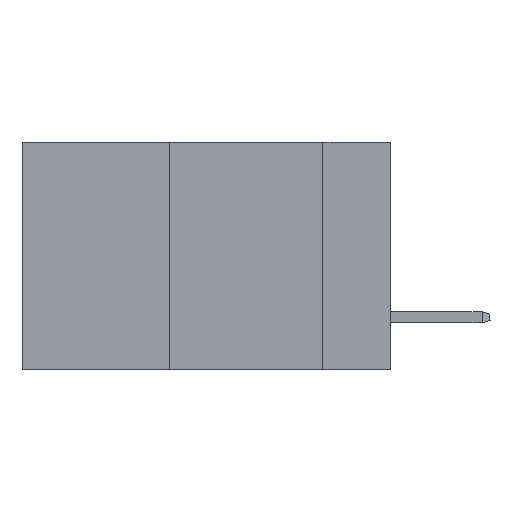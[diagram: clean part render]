
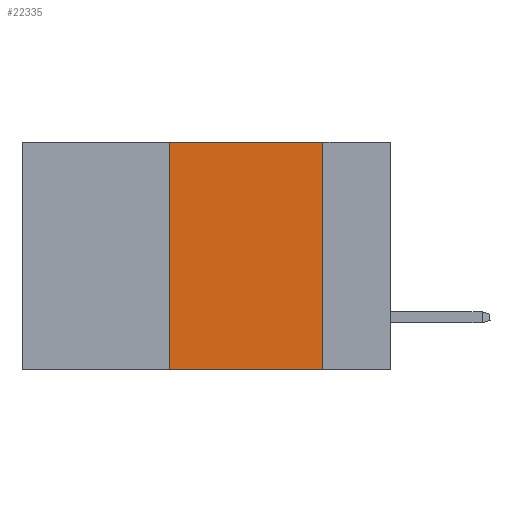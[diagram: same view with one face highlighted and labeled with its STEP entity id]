
A CAD part, left-side view. The second image highlights one B-rep face of the part: STEP entity #22335.
In plain terms, the highlighted planar face has unit normal (-1, 0, 0).
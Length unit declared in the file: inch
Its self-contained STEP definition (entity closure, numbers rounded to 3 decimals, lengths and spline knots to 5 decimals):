
#986 = VERTEX_POINT ( 'NONE', #29117 ) ;
#3581 = VECTOR ( 'NONE', #16260, 39.37008 ) ;
#5222 = DIRECTION ( 'NONE',  ( 0., 0., -1. ) ) ;
#5368 = CARTESIAN_POINT ( 'NONE',  ( 0., 0.11, 0. ) ) ;
#5947 = EDGE_CURVE ( 'NONE', #16020, #986, #28462, .T. ) ;
#6616 = LINE ( 'NONE', #5368, #40071 ) ;
#7700 = VECTOR ( 'NONE', #8585, 39.37008 ) ;
#8439 = CARTESIAN_POINT ( 'NONE',  ( 0., 0.6, -0.37 ) ) ;
#8585 = DIRECTION ( 'NONE',  ( 0., -1., 0. ) ) ;
#8957 = DIRECTION ( 'NONE',  ( 0., 0., -1. ) ) ;
#9080 = LINE ( 'NONE', #23895, #3581 ) ;
#10330 = DIRECTION ( 'NONE',  ( 0., 0., 1. ) ) ;
#10944 = VERTEX_POINT ( 'NONE', #11338 ) ;
#11338 = CARTESIAN_POINT ( 'NONE',  ( 0., 0.11, 0. ) ) ;
#11544 = ORIENTED_EDGE ( 'NONE', *, *, #27147, .T. ) ;
#12960 = CARTESIAN_POINT ( 'NONE',  ( 0., 0.36, 0. ) ) ;
#13044 = ORIENTED_EDGE ( 'NONE', *, *, #45331, .F. ) ;
#14497 = CARTESIAN_POINT ( 'NONE',  ( 0., 0.11, -0.37 ) ) ;
#15393 = CARTESIAN_POINT ( 'NONE',  ( 0., 0.36, -0.37 ) ) ;
#15721 = PLANE ( 'NONE',  #26505 ) ;
#16020 = VERTEX_POINT ( 'NONE', #15393 ) ;
#16260 = DIRECTION ( 'NONE',  ( 0., -1., 0. ) ) ;
#17795 = ORIENTED_EDGE ( 'NONE', *, *, #5947, .F. ) ;
#19452 = ORIENTED_EDGE ( 'NONE', *, *, #42508, .F. ) ;
#22335 = ADVANCED_FACE ( 'NONE', ( #39774 ), #15721, .F. ) ;
#23895 = CARTESIAN_POINT ( 'NONE',  ( 0., 0.6, 0. ) ) ;
#25799 = EDGE_LOOP ( 'NONE', ( #19452, #13044, #17795, #11544 ) ) ;
#26505 = AXIS2_PLACEMENT_3D ( 'NONE', #33462, #32873, #8957 ) ;
#27147 = EDGE_CURVE ( 'NONE', #16020, #36946, #37866, .T. ) ;
#28462 = LINE ( 'NONE', #12960, #34491 ) ;
#29117 = CARTESIAN_POINT ( 'NONE',  ( 0., 0.36, 0. ) ) ;
#32873 = DIRECTION ( 'NONE',  ( 1., 0., 0. ) ) ;
#33462 = CARTESIAN_POINT ( 'NONE',  ( 0., 0.6, 0. ) ) ;
#34491 = VECTOR ( 'NONE', #10330, 39.37008 ) ;
#36946 = VERTEX_POINT ( 'NONE', #14497 ) ;
#37866 = LINE ( 'NONE', #8439, #7700 ) ;
#39774 = FACE_OUTER_BOUND ( 'NONE', #25799, .T. ) ;
#40071 = VECTOR ( 'NONE', #5222, 39.37008 ) ;
#42508 = EDGE_CURVE ( 'NONE', #10944, #36946, #6616, .T. ) ;
#45331 = EDGE_CURVE ( 'NONE', #986, #10944, #9080, .T. ) ;
